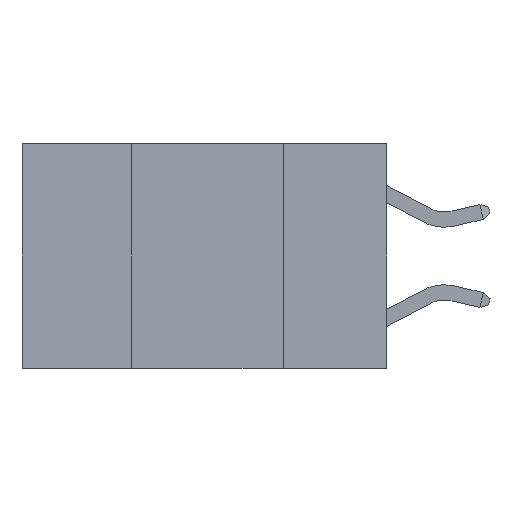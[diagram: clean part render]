
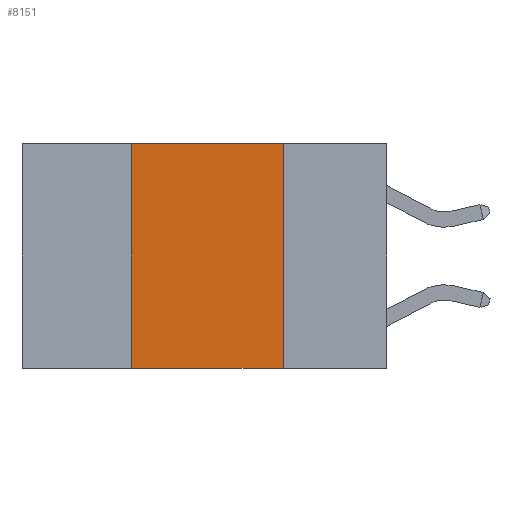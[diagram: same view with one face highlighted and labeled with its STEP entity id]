
A CAD part, left-side view. The second image highlights one B-rep face of the part: STEP entity #8151.
In plain terms, the highlighted planar face has unit normal (-1, 0, 0).
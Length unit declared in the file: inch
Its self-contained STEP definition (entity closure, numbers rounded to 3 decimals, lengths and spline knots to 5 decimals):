
#160 = FACE_OUTER_BOUND ( 'NONE', #5820, .T. ) ;
#370 = VERTEX_POINT ( 'NONE', #6819 ) ;
#487 = CARTESIAN_POINT ( 'NONE',  ( 0., 0.6, 0. ) ) ;
#533 = LINE ( 'NONE', #10024, #8647 ) ;
#572 = EDGE_CURVE ( 'NONE', #3427, #9012, #2979, .T. ) ;
#587 = ORIENTED_EDGE ( 'NONE', *, *, #8671, .F. ) ;
#1302 = DIRECTION ( 'NONE',  ( 0., 0., -1. ) ) ;
#1329 = ORIENTED_EDGE ( 'NONE', *, *, #572, .F. ) ;
#1710 = CARTESIAN_POINT ( 'NONE',  ( 0., 0.17, -0.37 ) ) ;
#2438 = ORIENTED_EDGE ( 'NONE', *, *, #8489, .T. ) ;
#2516 = VECTOR ( 'NONE', #4369, 39.37008 ) ;
#2574 = CARTESIAN_POINT ( 'NONE',  ( 0., 0.42, 0. ) ) ;
#2979 = LINE ( 'NONE', #8687, #4814 ) ;
#3228 = CARTESIAN_POINT ( 'NONE',  ( 0., 0.42, -0.37 ) ) ;
#3427 = VERTEX_POINT ( 'NONE', #3228 ) ;
#3922 = ORIENTED_EDGE ( 'NONE', *, *, #5925, .F. ) ;
#4028 = DIRECTION ( 'NONE',  ( 0., 0., 1. ) ) ;
#4357 = LINE ( 'NONE', #9820, #2516 ) ;
#4369 = DIRECTION ( 'NONE',  ( 0., -1., 0. ) ) ;
#4423 = PLANE ( 'NONE',  #7336 ) ;
#4814 = VECTOR ( 'NONE', #4028, 39.37008 ) ;
#5820 = EDGE_LOOP ( 'NONE', ( #587, #3922, #1329, #2438 ) ) ;
#5925 = EDGE_CURVE ( 'NONE', #9012, #370, #9655, .T. ) ;
#5992 = DIRECTION ( 'NONE',  ( 1., 0., 0. ) ) ;
#6143 = DIRECTION ( 'NONE',  ( 0., 0., -1. ) ) ;
#6819 = CARTESIAN_POINT ( 'NONE',  ( 0., 0.17, 0. ) ) ;
#7138 = DIRECTION ( 'NONE',  ( 0., -1., 0. ) ) ;
#7336 = AXIS2_PLACEMENT_3D ( 'NONE', #487, #5992, #1302 ) ;
#7605 = VECTOR ( 'NONE', #7138, 39.37008 ) ;
#8151 = ADVANCED_FACE ( 'NONE', ( #160 ), #4423, .F. ) ;
#8489 = EDGE_CURVE ( 'NONE', #3427, #10158, #4357, .T. ) ;
#8647 = VECTOR ( 'NONE', #6143, 39.37008 ) ;
#8671 = EDGE_CURVE ( 'NONE', #370, #10158, #533, .T. ) ;
#8687 = CARTESIAN_POINT ( 'NONE',  ( 0., 0.42, 0. ) ) ;
#8731 = CARTESIAN_POINT ( 'NONE',  ( 0., 0.6, 0. ) ) ;
#9012 = VERTEX_POINT ( 'NONE', #2574 ) ;
#9655 = LINE ( 'NONE', #8731, #7605 ) ;
#9820 = CARTESIAN_POINT ( 'NONE',  ( 0., 0.6, -0.37 ) ) ;
#10024 = CARTESIAN_POINT ( 'NONE',  ( 0., 0.17, 0. ) ) ;
#10158 = VERTEX_POINT ( 'NONE', #1710 ) ;
